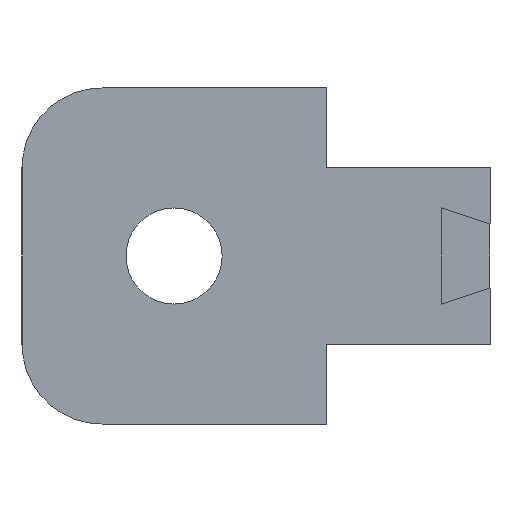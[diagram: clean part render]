
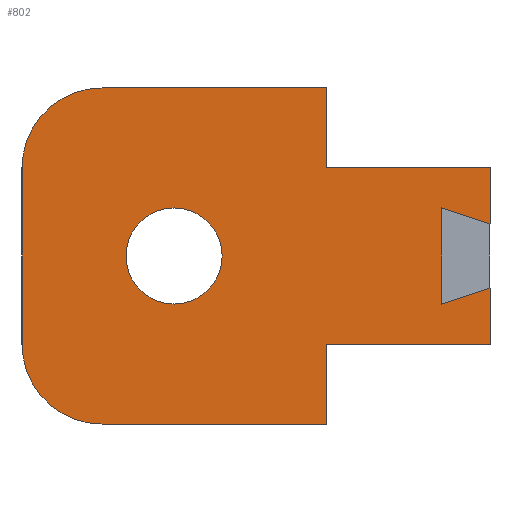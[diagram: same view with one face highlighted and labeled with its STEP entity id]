
A CAD part, left-side view. The second image highlights one B-rep face of the part: STEP entity #802.
In plain terms, the highlighted planar face has unit normal (-1, 0, 0).
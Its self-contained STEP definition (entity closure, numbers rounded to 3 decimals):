
#73=CARTESIAN_POINT('',(-27.006,-2.507,8.5));
#74=VERTEX_POINT('',#73);
#75=CARTESIAN_POINT('',(-27.006,-5.507,7.5));
#76=VERTEX_POINT('',#75);
#77=CARTESIAN_POINT('',(-27.006,-2.507,8.5));
#78=DIRECTION('',(0.,-0.949,-0.316));
#79=VECTOR('',#78,3.162);
#80=LINE('',#77,#79);
#81=EDGE_CURVE('',#74,#76,#80,.T.);
#113=CARTESIAN_POINT('',(-27.006,-2.507,2.5));
#114=VERTEX_POINT('',#113);
#115=CARTESIAN_POINT('',(-27.006,-2.507,2.5));
#116=DIRECTION('',(0.0,0.0,1.0));
#117=VECTOR('',#116,6.0);
#118=LINE('',#115,#117);
#119=EDGE_CURVE('',#114,#74,#118,.T.);
#144=CARTESIAN_POINT('',(-27.006,-5.507,3.5));
#145=VERTEX_POINT('',#144);
#146=CARTESIAN_POINT('',(-27.006,-5.507,3.5));
#147=DIRECTION('',(0.,0.949,-0.316));
#148=VECTOR('',#147,3.162);
#149=LINE('',#146,#148);
#150=EDGE_CURVE('',#145,#114,#149,.T.);
#195=CARTESIAN_POINT('',(-27.006,-5.507,0.0));
#196=VERTEX_POINT('',#195);
#197=CARTESIAN_POINT('',(-27.006,-5.507,0.0));
#198=DIRECTION('',(0.0,0.0,1.0));
#199=VECTOR('',#198,3.5);
#200=LINE('',#197,#199);
#201=EDGE_CURVE('',#196,#145,#200,.T.);
#219=CARTESIAN_POINT('',(-27.006,-5.507,11.0));
#220=VERTEX_POINT('',#219);
#227=CARTESIAN_POINT('',(-27.006,-5.507,7.5));
#228=DIRECTION('',(0.0,0.0,1.0));
#229=VECTOR('',#228,3.5);
#230=LINE('',#227,#229);
#231=EDGE_CURVE('',#76,#220,#230,.T.);
#418=CARTESIAN_POINT('',(-27.006,4.729,-5.0));
#419=VERTEX_POINT('',#418);
#426=CARTESIAN_POINT('',(-27.006,18.729,-5.0));
#427=VERTEX_POINT('',#426);
#428=CARTESIAN_POINT('',(-27.006,4.729,-5.0));
#429=DIRECTION('',(0.0,1.0,0.0));
#430=VECTOR('',#429,14.);
#431=LINE('',#428,#430);
#432=EDGE_CURVE('',#419,#427,#431,.T.);
#523=CARTESIAN_POINT('',(-27.006,4.729,0.0));
#524=VERTEX_POINT('',#523);
#531=CARTESIAN_POINT('',(-27.006,4.729,0.0));
#532=DIRECTION('',(0.0,0.0,-1.0));
#533=VECTOR('',#532,5.0);
#534=LINE('',#531,#533);
#535=EDGE_CURVE('',#524,#419,#534,.T.);
#546=CARTESIAN_POINT('',(-27.006,14.229,2.5));
#547=VERTEX_POINT('',#546);
#548=CARTESIAN_POINT('',(-27.006,14.229,5.5));
#549=DIRECTION('',(1.0,0.0,0.0));
#550=DIRECTION('',(0.0,0.0,1.0));
#551=AXIS2_PLACEMENT_3D('',#548,#549,#550);
#552=CIRCLE('',#551,3.0);
#553=EDGE_CURVE('',#547,#547,#552,.T.);
#567=CARTESIAN_POINT('',(-27.006,23.729,11.));
#568=VERTEX_POINT('',#567);
#575=CARTESIAN_POINT('',(-27.006,18.729,16.0));
#576=VERTEX_POINT('',#575);
#577=CARTESIAN_POINT('',(-27.006,18.729,11.));
#578=DIRECTION('',(1.0,0.,0.));
#579=DIRECTION('',(0.,0.707,0.707));
#580=AXIS2_PLACEMENT_3D('',#577,#578,#579);
#581=CIRCLE('',#580,5.);
#582=EDGE_CURVE('',#568,#576,#581,.T.);
#600=CARTESIAN_POINT('',(-27.006,23.729,0.0));
#601=VERTEX_POINT('',#600);
#608=CARTESIAN_POINT('',(-27.006,23.729,0.0));
#609=DIRECTION('',(0.0,0.0,1.0));
#610=VECTOR('',#609,11.);
#611=LINE('',#608,#610);
#612=EDGE_CURVE('',#601,#568,#611,.T.);
#624=CARTESIAN_POINT('',(-27.006,18.729,0.0));
#625=DIRECTION('',(1.0,0.,0.));
#626=DIRECTION('',(0.,0.707,-0.707));
#627=AXIS2_PLACEMENT_3D('',#624,#625,#626);
#628=CIRCLE('',#627,5.0);
#629=EDGE_CURVE('',#427,#601,#628,.T.);
#641=CARTESIAN_POINT('',(-27.006,4.729,16.0));
#642=VERTEX_POINT('',#641);
#649=CARTESIAN_POINT('',(-27.006,4.729,11.0));
#650=VERTEX_POINT('',#649);
#651=CARTESIAN_POINT('',(-27.006,4.729,11.0));
#652=DIRECTION('',(0.0,0.0,1.0));
#653=VECTOR('',#652,5.0);
#654=LINE('',#651,#653);
#655=EDGE_CURVE('',#650,#642,#654,.T.);
#674=CARTESIAN_POINT('',(-27.006,18.729,16.0));
#675=DIRECTION('',(0.0,-1.0,0.0));
#676=VECTOR('',#675,14.0);
#677=LINE('',#674,#676);
#678=EDGE_CURVE('',#576,#642,#677,.T.);
#768=CARTESIAN_POINT('',(-27.006,23.729,0.0));
#769=DIRECTION('',(-1.0,0.0,0.0));
#770=DIRECTION('',(0.0,-1.0,0.0));
#771=AXIS2_PLACEMENT_3D('',#768,#769,#770);
#772=PLANE('',#771);
#773=ORIENTED_EDGE('',*,*,#81,.T.);
#774=ORIENTED_EDGE('',*,*,#231,.T.);
#775=CARTESIAN_POINT('',(-27.006,4.729,11.0));
#776=DIRECTION('',(0.0,-1.0,0.0));
#777=VECTOR('',#776,10.235);
#778=LINE('',#775,#777);
#779=EDGE_CURVE('',#650,#220,#778,.T.);
#780=ORIENTED_EDGE('',*,*,#779,.F.);
#781=ORIENTED_EDGE('',*,*,#655,.T.);
#782=ORIENTED_EDGE('',*,*,#678,.F.);
#783=ORIENTED_EDGE('',*,*,#582,.F.);
#784=ORIENTED_EDGE('',*,*,#612,.F.);
#785=ORIENTED_EDGE('',*,*,#629,.F.);
#786=ORIENTED_EDGE('',*,*,#432,.F.);
#787=ORIENTED_EDGE('',*,*,#535,.F.);
#788=CARTESIAN_POINT('',(-27.006,-5.507,0.0));
#789=DIRECTION('',(0.0,1.0,0.0));
#790=VECTOR('',#789,10.235);
#791=LINE('',#788,#790);
#792=EDGE_CURVE('',#196,#524,#791,.T.);
#793=ORIENTED_EDGE('',*,*,#792,.F.);
#794=ORIENTED_EDGE('',*,*,#201,.T.);
#795=ORIENTED_EDGE('',*,*,#150,.T.);
#796=ORIENTED_EDGE('',*,*,#119,.T.);
#797=EDGE_LOOP('',(#773,#774,#780,#781,#782,#783,#784,#785,#786,#787,#793,#794,#795,#796));
#798=FACE_OUTER_BOUND('',#797,.T.);
#799=ORIENTED_EDGE('',*,*,#553,.T.);
#800=EDGE_LOOP('',(#799));
#801=FACE_BOUND('',#800,.T.);
#802=ADVANCED_FACE('',(#798,#801),#772,.T.);
